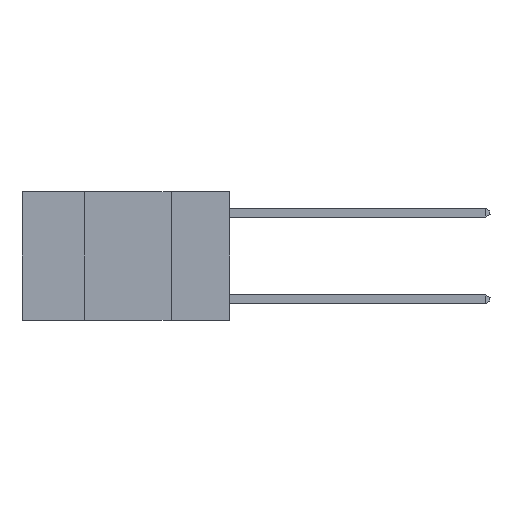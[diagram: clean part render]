
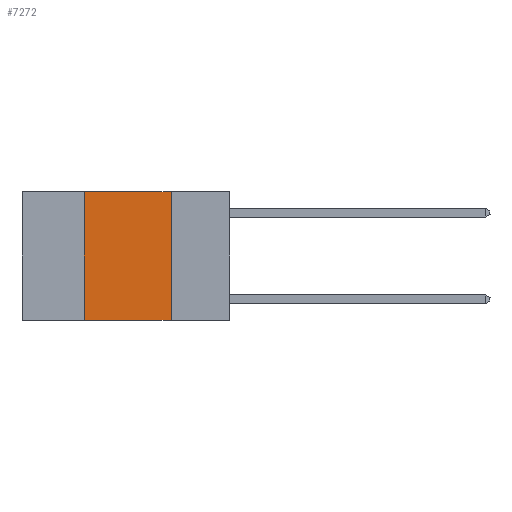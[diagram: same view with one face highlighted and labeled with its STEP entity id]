
A CAD part, left-side view. The second image highlights one B-rep face of the part: STEP entity #7272.
In plain terms, the highlighted planar face has unit normal (-1, 0, 0).
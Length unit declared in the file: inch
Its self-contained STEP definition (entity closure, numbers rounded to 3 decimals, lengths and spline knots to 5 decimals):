
#352 = VERTEX_POINT ( 'NONE', #8325 ) ;
#556 = LINE ( 'NONE', #1923, #3576 ) ;
#1074 = CARTESIAN_POINT ( 'NONE',  ( 0., 0.17, 0. ) ) ;
#1544 = LINE ( 'NONE', #1708, #13904 ) ;
#1708 = CARTESIAN_POINT ( 'NONE',  ( 0., 0.6, 0. ) ) ;
#1923 = CARTESIAN_POINT ( 'NONE',  ( 0., 0.6, -0.37 ) ) ;
#2995 = LINE ( 'NONE', #4461, #15220 ) ;
#3166 = DIRECTION ( 'NONE',  ( 0., 0., -1. ) ) ;
#3576 = VECTOR ( 'NONE', #14969, 39.37008 ) ;
#4458 = PLANE ( 'NONE',  #13599 ) ;
#4461 = CARTESIAN_POINT ( 'NONE',  ( 0., 0.42, 0. ) ) ;
#4485 = CARTESIAN_POINT ( 'NONE',  ( 0., 0.17, -0.37 ) ) ;
#4779 = VERTEX_POINT ( 'NONE', #4485 ) ;
#4785 = VERTEX_POINT ( 'NONE', #6959 ) ;
#5026 = ORIENTED_EDGE ( 'NONE', *, *, #11879, .F. ) ;
#5110 = DIRECTION ( 'NONE',  ( 0., 0., -1. ) ) ;
#6354 = ORIENTED_EDGE ( 'NONE', *, *, #11127, .F. ) ;
#6393 = ORIENTED_EDGE ( 'NONE', *, *, #8467, .F. ) ;
#6624 = VERTEX_POINT ( 'NONE', #11901 ) ;
#6671 = EDGE_LOOP ( 'NONE', ( #6354, #5026, #6393, #14071 ) ) ;
#6850 = DIRECTION ( 'NONE',  ( 1., 0., 0. ) ) ;
#6959 = CARTESIAN_POINT ( 'NONE',  ( 0., 0.42, -0.37 ) ) ;
#7272 = ADVANCED_FACE ( 'NONE', ( #16124 ), #4458, .F. ) ;
#7894 = VECTOR ( 'NONE', #5110, 39.37008 ) ;
#8325 = CARTESIAN_POINT ( 'NONE',  ( 0., 0.17, 0. ) ) ;
#8467 = EDGE_CURVE ( 'NONE', #4785, #6624, #2995, .T. ) ;
#9607 = DIRECTION ( 'NONE',  ( 0., -1., 0. ) ) ;
#9686 = CARTESIAN_POINT ( 'NONE',  ( 0., 0.6, 0. ) ) ;
#9689 = DIRECTION ( 'NONE',  ( 0., 0., 1. ) ) ;
#11127 = EDGE_CURVE ( 'NONE', #352, #4779, #14102, .T. ) ;
#11879 = EDGE_CURVE ( 'NONE', #6624, #352, #1544, .T. ) ;
#11901 = CARTESIAN_POINT ( 'NONE',  ( 0., 0.42, 0. ) ) ;
#12389 = EDGE_CURVE ( 'NONE', #4785, #4779, #556, .T. ) ;
#13599 = AXIS2_PLACEMENT_3D ( 'NONE', #9686, #6850, #3166 ) ;
#13904 = VECTOR ( 'NONE', #9607, 39.37008 ) ;
#14071 = ORIENTED_EDGE ( 'NONE', *, *, #12389, .T. ) ;
#14102 = LINE ( 'NONE', #1074, #7894 ) ;
#14969 = DIRECTION ( 'NONE',  ( 0., -1., 0. ) ) ;
#15220 = VECTOR ( 'NONE', #9689, 39.37008 ) ;
#16124 = FACE_OUTER_BOUND ( 'NONE', #6671, .T. ) ;
